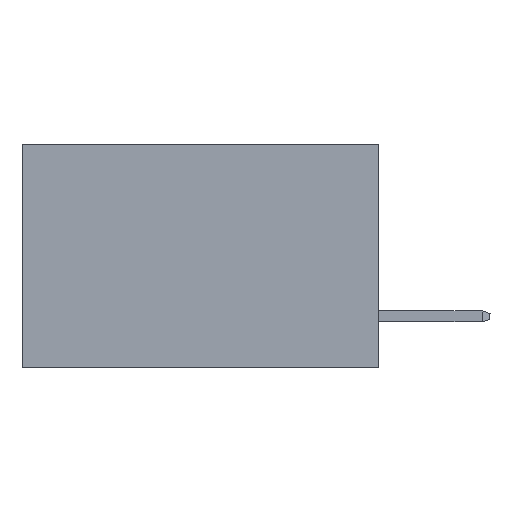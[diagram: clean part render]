
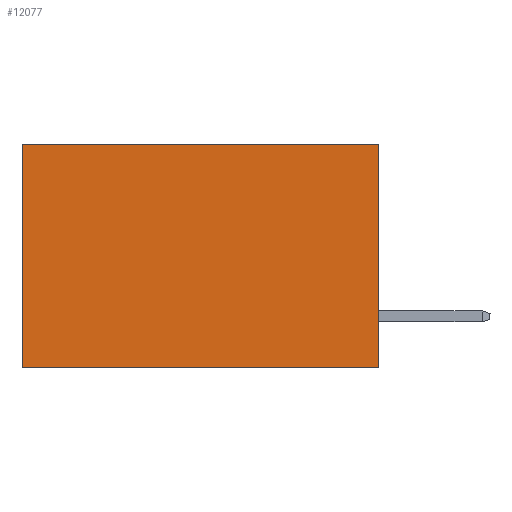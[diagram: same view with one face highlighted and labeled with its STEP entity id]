
A CAD part, left-side view. The second image highlights one B-rep face of the part: STEP entity #12077.
In plain terms, the highlighted planar face has unit normal (-1, 0, 0).
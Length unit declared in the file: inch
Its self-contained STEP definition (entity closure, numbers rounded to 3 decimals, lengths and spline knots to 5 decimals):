
#77 = AXIS2_PLACEMENT_3D ( 'NONE', #10362, #3995, #12816 ) ;
#1054 = ORIENTED_EDGE ( 'NONE', *, *, #8767, .T. ) ;
#1559 = CARTESIAN_POINT ( 'NONE',  ( 0.277, 0., 0. ) ) ;
#1664 = VERTEX_POINT ( 'NONE', #5800 ) ;
#1696 = EDGE_LOOP ( 'NONE', ( #1054, #11742, #11991, #5305 ) ) ;
#2141 = EDGE_CURVE ( 'NONE', #15565, #6639, #6170, .T. ) ;
#2754 = PLANE ( 'NONE',  #77 ) ;
#2782 = VECTOR ( 'NONE', #10662, 39.37008 ) ;
#3102 = DIRECTION ( 'NONE',  ( 0., 1., 0. ) ) ;
#3268 = CARTESIAN_POINT ( 'NONE',  ( 0.277, 0., -0.37 ) ) ;
#3832 = CARTESIAN_POINT ( 'NONE',  ( 0.277, 0.59, -0.37 ) ) ;
#3922 = DIRECTION ( 'NONE',  ( 0., 0., -1. ) ) ;
#3995 = DIRECTION ( 'NONE',  ( 1., 0., 0. ) ) ;
#4671 = CARTESIAN_POINT ( 'NONE',  ( 0.277, 0., 0. ) ) ;
#5148 = LINE ( 'NONE', #3268, #14315 ) ;
#5305 = ORIENTED_EDGE ( 'NONE', *, *, #2141, .T. ) ;
#5800 = CARTESIAN_POINT ( 'NONE',  ( 0.277, 0., -0.37 ) ) ;
#6006 = VECTOR ( 'NONE', #3922, 39.37008 ) ;
#6086 = VERTEX_POINT ( 'NONE', #15255 ) ;
#6170 = LINE ( 'NONE', #1559, #2782 ) ;
#6639 = VERTEX_POINT ( 'NONE', #11032 ) ;
#8767 = EDGE_CURVE ( 'NONE', #6639, #6086, #11899, .T. ) ;
#9591 = DIRECTION ( 'NONE',  ( 0., 0., -1. ) ) ;
#9644 = CARTESIAN_POINT ( 'NONE',  ( 0.277, 0., -0.37 ) ) ;
#9719 = VECTOR ( 'NONE', #9591, 39.37008 ) ;
#10362 = CARTESIAN_POINT ( 'NONE',  ( 0.277, 0., -0.37 ) ) ;
#10512 = FACE_OUTER_BOUND ( 'NONE', #1696, .T. ) ;
#10629 = EDGE_CURVE ( 'NONE', #15565, #1664, #12996, .T. ) ;
#10662 = DIRECTION ( 'NONE',  ( 0., 1., 0. ) ) ;
#11032 = CARTESIAN_POINT ( 'NONE',  ( 0.277, 0.59, 0. ) ) ;
#11203 = EDGE_CURVE ( 'NONE', #1664, #6086, #5148, .T. ) ;
#11742 = ORIENTED_EDGE ( 'NONE', *, *, #11203, .F. ) ;
#11899 = LINE ( 'NONE', #3832, #6006 ) ;
#11991 = ORIENTED_EDGE ( 'NONE', *, *, #10629, .F. ) ;
#12077 = ADVANCED_FACE ( 'NONE', ( #10512 ), #2754, .F. ) ;
#12816 = DIRECTION ( 'NONE',  ( 0., 0., -1. ) ) ;
#12996 = LINE ( 'NONE', #9644, #9719 ) ;
#14315 = VECTOR ( 'NONE', #3102, 39.37008 ) ;
#15255 = CARTESIAN_POINT ( 'NONE',  ( 0.277, 0.59, -0.37 ) ) ;
#15565 = VERTEX_POINT ( 'NONE', #4671 ) ;
